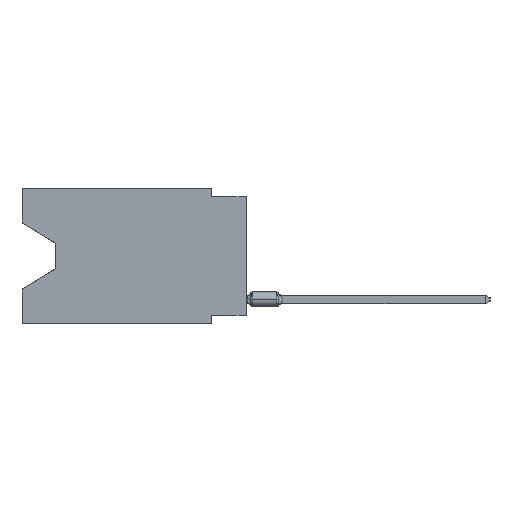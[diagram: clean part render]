
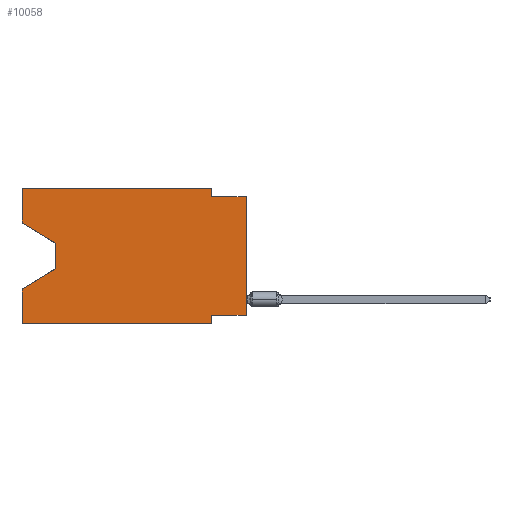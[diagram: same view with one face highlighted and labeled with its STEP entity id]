
A CAD part, left-side view. The second image highlights one B-rep face of the part: STEP entity #10058.
In plain terms, the highlighted planar face has unit normal (-1, 0, 0).
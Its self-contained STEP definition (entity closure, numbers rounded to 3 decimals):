
#646 = ORIENTED_EDGE ( 'NONE', *, *, #61933, .F. ) ;
#1268 = ORIENTED_EDGE ( 'NONE', *, *, #19259, .T. ) ;
#1995 = EDGE_CURVE ( 'NONE', #59408, #14020, #48407, .T. ) ;
#3978 = LINE ( 'NONE', #17767, #47970 ) ;
#4434 = VECTOR ( 'NONE', #23720, 1000. ) ;
#4663 = LINE ( 'NONE', #30966, #28788 ) ;
#5306 = LINE ( 'NONE', #36839, #18198 ) ;
#6393 = VERTEX_POINT ( 'NONE', #29262 ) ;
#8691 = VECTOR ( 'NONE', #26358, 1000. ) ;
#9985 = VERTEX_POINT ( 'NONE', #23409 ) ;
#10058 = ADVANCED_FACE ( 'NONE', ( #18185 ), #24666, .F. ) ;
#10223 = DIRECTION ( 'NONE',  ( 0., 0., 1. ) ) ;
#11177 = LINE ( 'NONE', #17251, #4434 ) ;
#11259 = LINE ( 'NONE', #71695, #64910 ) ;
#12980 = EDGE_CURVE ( 'NONE', #55426, #39153, #5306, .T. ) ;
#14020 = VERTEX_POINT ( 'NONE', #44402 ) ;
#14125 = CARTESIAN_POINT ( 'NONE',  ( 0., 16.383, -9.906 ) ) ;
#14847 = VECTOR ( 'NONE', #31125, 1000. ) ;
#14982 = DIRECTION ( 'NONE',  ( 0., 0., -1. ) ) ;
#16336 = DIRECTION ( 'NONE',  ( 0., 0., 1. ) ) ;
#17251 = CARTESIAN_POINT ( 'NONE',  ( 0., 16.383, -2.546 ) ) ;
#17767 = CARTESIAN_POINT ( 'NONE',  ( 0., 13.97, -5.893 ) ) ;
#18185 = FACE_OUTER_BOUND ( 'NONE', #57779, .T. ) ;
#18198 = VECTOR ( 'NONE', #70947, 1000. ) ;
#19242 = EDGE_CURVE ( 'NONE', #32819, #82983, #76546, .T. ) ;
#19259 = EDGE_CURVE ( 'NONE', #39153, #6393, #3978, .T. ) ;
#19406 = LINE ( 'NONE', #51813, #80874 ) ;
#19449 = LINE ( 'NONE', #72159, #8691 ) ;
#21550 = CARTESIAN_POINT ( 'NONE',  ( 0., 16.383, 0. ) ) ;
#23340 = VECTOR ( 'NONE', #10223, 1000. ) ;
#23409 = CARTESIAN_POINT ( 'NONE',  ( 0., 2.54, -0.635 ) ) ;
#23616 = VECTOR ( 'NONE', #14982, 1000. ) ;
#23720 = DIRECTION ( 'NONE',  ( 0., -0.855, -0.519 ) ) ;
#24666 = PLANE ( 'NONE',  #33013 ) ;
#25338 = ORIENTED_EDGE ( 'NONE', *, *, #32712, .F. ) ;
#25937 = DIRECTION ( 'NONE',  ( 0., 0., -1. ) ) ;
#26358 = DIRECTION ( 'NONE',  ( 0., 1., 0. ) ) ;
#28018 = LINE ( 'NONE', #21550, #29785 ) ;
#28226 = ORIENTED_EDGE ( 'NONE', *, *, #66918, .F. ) ;
#28788 = VECTOR ( 'NONE', #16336, 1000. ) ;
#29262 = CARTESIAN_POINT ( 'NONE',  ( 0., 16.383, -7.36 ) ) ;
#29289 = DIRECTION ( 'NONE',  ( 0., -1., 0. ) ) ;
#29760 = ORIENTED_EDGE ( 'NONE', *, *, #12980, .T. ) ;
#29785 = VECTOR ( 'NONE', #29289, 1000. ) ;
#30707 = VERTEX_POINT ( 'NONE', #40372 ) ;
#30966 = CARTESIAN_POINT ( 'NONE',  ( 0., 16.383, 0. ) ) ;
#31125 = DIRECTION ( 'NONE',  ( 0., 0., -1. ) ) ;
#31537 = ORIENTED_EDGE ( 'NONE', *, *, #80341, .T. ) ;
#32712 = EDGE_CURVE ( 'NONE', #9985, #14020, #11259, .T. ) ;
#32819 = VERTEX_POINT ( 'NONE', #73414 ) ;
#33013 = AXIS2_PLACEMENT_3D ( 'NONE', #51025, #71311, #25937 ) ;
#33200 = ORIENTED_EDGE ( 'NONE', *, *, #71007, .F. ) ;
#33471 = EDGE_CURVE ( 'NONE', #70725, #6393, #43455, .T. ) ;
#33708 = CARTESIAN_POINT ( 'NONE',  ( 0., 0., 0. ) ) ;
#36120 = LINE ( 'NONE', #81905, #23616 ) ;
#36659 = VERTEX_POINT ( 'NONE', #82440 ) ;
#36839 = CARTESIAN_POINT ( 'NONE',  ( 0., 13.97, -4.013 ) ) ;
#37196 = CARTESIAN_POINT ( 'NONE',  ( 0., 2.54, -9.906 ) ) ;
#39153 = VERTEX_POINT ( 'NONE', #44480 ) ;
#39994 = ORIENTED_EDGE ( 'NONE', *, *, #45062, .T. ) ;
#40372 = CARTESIAN_POINT ( 'NONE',  ( 0., 2.54, 0. ) ) ;
#42111 = CARTESIAN_POINT ( 'NONE',  ( 0., 0., -9.271 ) ) ;
#43455 = LINE ( 'NONE', #83609, #23340 ) ;
#44402 = CARTESIAN_POINT ( 'NONE',  ( 0., 0., -0.635 ) ) ;
#44480 = CARTESIAN_POINT ( 'NONE',  ( 0., 13.97, -5.893 ) ) ;
#45062 = EDGE_CURVE ( 'NONE', #36659, #55426, #11177, .T. ) ;
#45701 = CARTESIAN_POINT ( 'NONE',  ( 0., 2.54, -9.906 ) ) ;
#47970 = VECTOR ( 'NONE', #51018, 1000. ) ;
#47977 = DIRECTION ( 'NONE',  ( 0., 0., 1. ) ) ;
#48407 = LINE ( 'NONE', #33708, #50907 ) ;
#50907 = VECTOR ( 'NONE', #47977, 1000. ) ;
#51018 = DIRECTION ( 'NONE',  ( 0., 0.855, -0.519 ) ) ;
#51025 = CARTESIAN_POINT ( 'NONE',  ( 0., 16.383, 0. ) ) ;
#51813 = CARTESIAN_POINT ( 'NONE',  ( 0., 16.383, -9.906 ) ) ;
#54532 = ORIENTED_EDGE ( 'NONE', *, *, #33471, .F. ) ;
#55426 = VERTEX_POINT ( 'NONE', #65722 ) ;
#57779 = EDGE_LOOP ( 'NONE', ( #39994, #29760, #1268, #54532, #31537, #68544, #33200, #69918, #25338, #28226, #646, #84308 ) ) ;
#59408 = VERTEX_POINT ( 'NONE', #42111 ) ;
#61933 = EDGE_CURVE ( 'NONE', #76327, #30707, #28018, .T. ) ;
#62076 = EDGE_CURVE ( 'NONE', #36659, #76327, #4663, .T. ) ;
#64910 = VECTOR ( 'NONE', #70844, 1000. ) ;
#65199 = DIRECTION ( 'NONE',  ( 0., -1., 0. ) ) ;
#65722 = CARTESIAN_POINT ( 'NONE',  ( 0., 13.97, -4.013 ) ) ;
#66918 = EDGE_CURVE ( 'NONE', #30707, #9985, #36120, .T. ) ;
#68544 = ORIENTED_EDGE ( 'NONE', *, *, #19242, .F. ) ;
#69918 = ORIENTED_EDGE ( 'NONE', *, *, #1995, .T. ) ;
#70725 = VERTEX_POINT ( 'NONE', #14125 ) ;
#70844 = DIRECTION ( 'NONE',  ( 0., -1., 0. ) ) ;
#70947 = DIRECTION ( 'NONE',  ( 0., 0., -1. ) ) ;
#71007 = EDGE_CURVE ( 'NONE', #59408, #32819, #19449, .T. ) ;
#71311 = DIRECTION ( 'NONE',  ( 1., 0., 0. ) ) ;
#71695 = CARTESIAN_POINT ( 'NONE',  ( 0., 0., -0.635 ) ) ;
#72159 = CARTESIAN_POINT ( 'NONE',  ( 0., 0., -9.271 ) ) ;
#73414 = CARTESIAN_POINT ( 'NONE',  ( 0., 2.54, -9.271 ) ) ;
#76327 = VERTEX_POINT ( 'NONE', #79405 ) ;
#76546 = LINE ( 'NONE', #37196, #14847 ) ;
#79405 = CARTESIAN_POINT ( 'NONE',  ( 0., 16.383, 0. ) ) ;
#80341 = EDGE_CURVE ( 'NONE', #70725, #82983, #19406, .T. ) ;
#80874 = VECTOR ( 'NONE', #65199, 1000. ) ;
#81905 = CARTESIAN_POINT ( 'NONE',  ( 0., 2.54, 0. ) ) ;
#82440 = CARTESIAN_POINT ( 'NONE',  ( 0., 16.383, -2.546 ) ) ;
#82983 = VERTEX_POINT ( 'NONE', #45701 ) ;
#83609 = CARTESIAN_POINT ( 'NONE',  ( 0., 16.383, 0. ) ) ;
#84308 = ORIENTED_EDGE ( 'NONE', *, *, #62076, .F. ) ;
